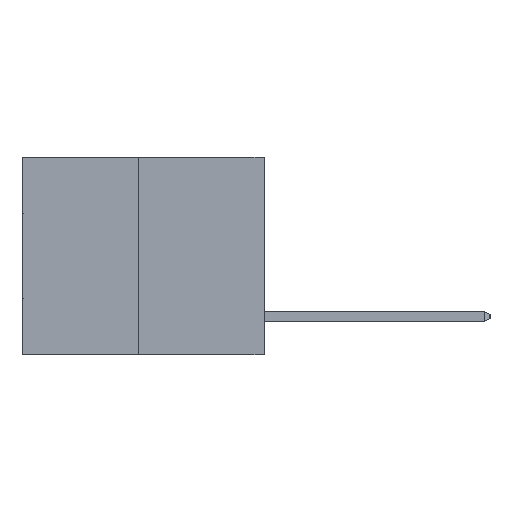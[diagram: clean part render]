
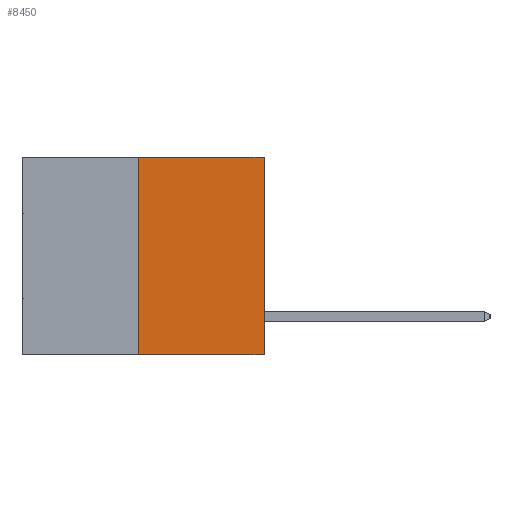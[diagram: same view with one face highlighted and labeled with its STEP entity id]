
A CAD part, left-side view. The second image highlights one B-rep face of the part: STEP entity #8450.
In plain terms, the highlighted planar face has unit normal (-1, 0, 0).
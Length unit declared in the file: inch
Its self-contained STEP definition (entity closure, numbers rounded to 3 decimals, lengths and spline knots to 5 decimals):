
#1120 = CARTESIAN_POINT ( 'NONE',  ( 0., 0.6, 0. ) ) ;
#1533 = EDGE_CURVE ( 'NONE', #25412, #31896, #13592, .T. ) ;
#2426 = CARTESIAN_POINT ( 'NONE',  ( 0., 0., 0. ) ) ;
#3771 = CARTESIAN_POINT ( 'NONE',  ( 0., 0.312, -0.49 ) ) ;
#3784 = LINE ( 'NONE', #9776, #6610 ) ;
#4970 = FACE_OUTER_BOUND ( 'NONE', #22964, .T. ) ;
#5118 = ORIENTED_EDGE ( 'NONE', *, *, #33151, .T. ) ;
#6275 = AXIS2_PLACEMENT_3D ( 'NONE', #1120, #6561, #11789 ) ;
#6561 = DIRECTION ( 'NONE',  ( 1., 0., 0. ) ) ;
#6610 = VECTOR ( 'NONE', #12265, 39.37008 ) ;
#6866 = VERTEX_POINT ( 'NONE', #3771 ) ;
#8105 = LINE ( 'NONE', #33615, #28451 ) ;
#8450 = ADVANCED_FACE ( 'NONE', ( #4970 ), #16681, .F. ) ;
#9301 = CARTESIAN_POINT ( 'NONE',  ( 0., 0., -0.49 ) ) ;
#9776 = CARTESIAN_POINT ( 'NONE',  ( 0., 0.312, -0.49 ) ) ;
#10331 = DIRECTION ( 'NONE',  ( 0., -1., 0. ) ) ;
#11789 = DIRECTION ( 'NONE',  ( 0., 0., -1. ) ) ;
#12265 = DIRECTION ( 'NONE',  ( 0., 0., 1. ) ) ;
#13592 = LINE ( 'NONE', #2426, #20950 ) ;
#13940 = ORIENTED_EDGE ( 'NONE', *, *, #26973, .F. ) ;
#16681 = PLANE ( 'NONE',  #6275 ) ;
#17720 = LINE ( 'NONE', #33580, #30279 ) ;
#19530 = VERTEX_POINT ( 'NONE', #22205 ) ;
#19914 = ORIENTED_EDGE ( 'NONE', *, *, #1533, .T. ) ;
#20610 = DIRECTION ( 'NONE',  ( 0., 0., 1. ) ) ;
#20706 = DIRECTION ( 'NONE',  ( 0., -1., 0. ) ) ;
#20950 = VECTOR ( 'NONE', #20610, 39.37008 ) ;
#22205 = CARTESIAN_POINT ( 'NONE',  ( 0., 0.312, 0. ) ) ;
#22964 = EDGE_LOOP ( 'NONE', ( #13940, #5118, #19914, #24840 ) ) ;
#24840 = ORIENTED_EDGE ( 'NONE', *, *, #25857, .F. ) ;
#25412 = VERTEX_POINT ( 'NONE', #9301 ) ;
#25857 = EDGE_CURVE ( 'NONE', #19530, #31896, #17720, .T. ) ;
#26973 = EDGE_CURVE ( 'NONE', #6866, #19530, #3784, .T. ) ;
#28451 = VECTOR ( 'NONE', #20706, 39.37008 ) ;
#30279 = VECTOR ( 'NONE', #10331, 39.37008 ) ;
#31896 = VERTEX_POINT ( 'NONE', #31931 ) ;
#31931 = CARTESIAN_POINT ( 'NONE',  ( 0., 0., 0. ) ) ;
#33151 = EDGE_CURVE ( 'NONE', #6866, #25412, #8105, .T. ) ;
#33580 = CARTESIAN_POINT ( 'NONE',  ( 0., 0.6, 0. ) ) ;
#33615 = CARTESIAN_POINT ( 'NONE',  ( 0., 0.6, -0.49 ) ) ;
